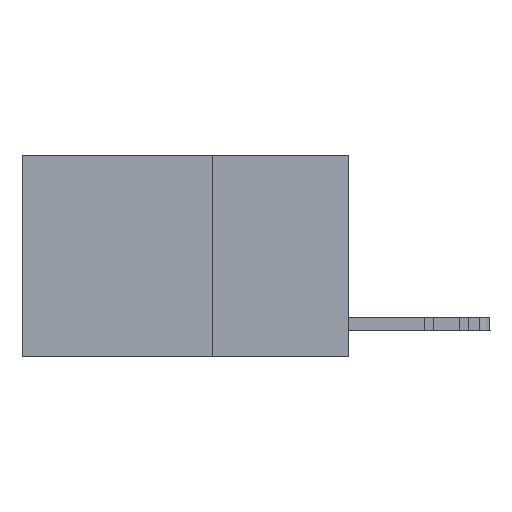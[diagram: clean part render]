
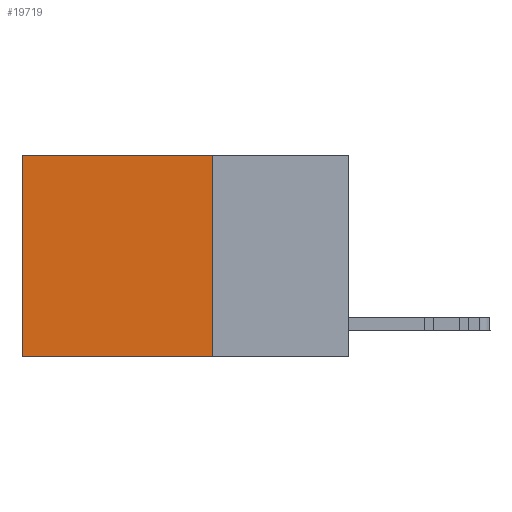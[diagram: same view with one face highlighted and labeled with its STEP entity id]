
A CAD part, left-side view. The second image highlights one B-rep face of the part: STEP entity #19719.
In plain terms, the highlighted planar face has unit normal (-1, 0, 0).
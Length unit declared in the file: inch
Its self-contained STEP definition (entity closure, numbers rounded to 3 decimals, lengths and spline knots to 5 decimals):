
#255 = LINE ( 'NONE', #19765, #13308 ) ;
#661 = DIRECTION ( 'NONE',  ( 0., 1., 0. ) ) ;
#2276 = CARTESIAN_POINT ( 'NONE',  ( 0.2625, 0.25, 0. ) ) ;
#3854 = DIRECTION ( 'NONE',  ( 0., 0., -1. ) ) ;
#3894 = CARTESIAN_POINT ( 'NONE',  ( 0.2625, 0.25, -0.37 ) ) ;
#4279 = EDGE_CURVE ( 'NONE', #11417, #8216, #27856, .T. ) ;
#4427 = FACE_OUTER_BOUND ( 'NONE', #18358, .T. ) ;
#5317 = EDGE_CURVE ( 'NONE', #9462, #26823, #27014, .T. ) ;
#6070 = CARTESIAN_POINT ( 'NONE',  ( 0.2625, 0.6, 0. ) ) ;
#6106 = EDGE_CURVE ( 'NONE', #9462, #11417, #255, .T. ) ;
#8134 = CARTESIAN_POINT ( 'NONE',  ( 0.2625, 0.6, 0. ) ) ;
#8216 = VERTEX_POINT ( 'NONE', #9701 ) ;
#8283 = VECTOR ( 'NONE', #661, 39.37008 ) ;
#9337 = DIRECTION ( 'NONE',  ( 0., 0., -1. ) ) ;
#9406 = DIRECTION ( 'NONE',  ( 0., 1., 0. ) ) ;
#9462 = VERTEX_POINT ( 'NONE', #11418 ) ;
#9701 = CARTESIAN_POINT ( 'NONE',  ( 0.2625, 0.6, -0.37 ) ) ;
#10033 = ORIENTED_EDGE ( 'NONE', *, *, #4279, .T. ) ;
#10271 = VECTOR ( 'NONE', #3854, 39.37008 ) ;
#10610 = ORIENTED_EDGE ( 'NONE', *, *, #5317, .F. ) ;
#11417 = VERTEX_POINT ( 'NONE', #6070 ) ;
#11418 = CARTESIAN_POINT ( 'NONE',  ( 0.2625, 0.25, 0. ) ) ;
#12041 = AXIS2_PLACEMENT_3D ( 'NONE', #2276, #21946, #17475 ) ;
#12572 = PLANE ( 'NONE',  #12041 ) ;
#13308 = VECTOR ( 'NONE', #9406, 39.37008 ) ;
#13490 = CARTESIAN_POINT ( 'NONE',  ( 0.2625, 0.25, 0. ) ) ;
#13689 = CARTESIAN_POINT ( 'NONE',  ( 0.2625, 0.25, -0.37 ) ) ;
#13987 = LINE ( 'NONE', #13689, #8283 ) ;
#14579 = VECTOR ( 'NONE', #9337, 39.37008 ) ;
#17437 = ORIENTED_EDGE ( 'NONE', *, *, #23505, .F. ) ;
#17475 = DIRECTION ( 'NONE',  ( 0., 0., -1. ) ) ;
#17646 = ORIENTED_EDGE ( 'NONE', *, *, #6106, .T. ) ;
#18358 = EDGE_LOOP ( 'NONE', ( #10033, #17437, #10610, #17646 ) ) ;
#19719 = ADVANCED_FACE ( 'NONE', ( #4427 ), #12572, .F. ) ;
#19765 = CARTESIAN_POINT ( 'NONE',  ( 0.2625, 0.25, 0. ) ) ;
#21946 = DIRECTION ( 'NONE',  ( 1., 0., 0. ) ) ;
#23505 = EDGE_CURVE ( 'NONE', #26823, #8216, #13987, .T. ) ;
#26823 = VERTEX_POINT ( 'NONE', #3894 ) ;
#27014 = LINE ( 'NONE', #13490, #14579 ) ;
#27856 = LINE ( 'NONE', #8134, #10271 ) ;
